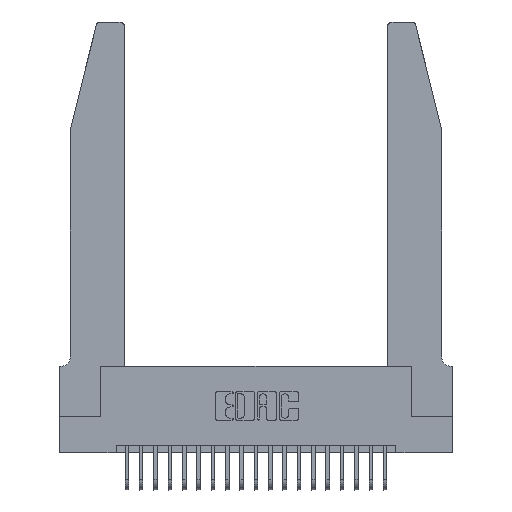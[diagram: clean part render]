
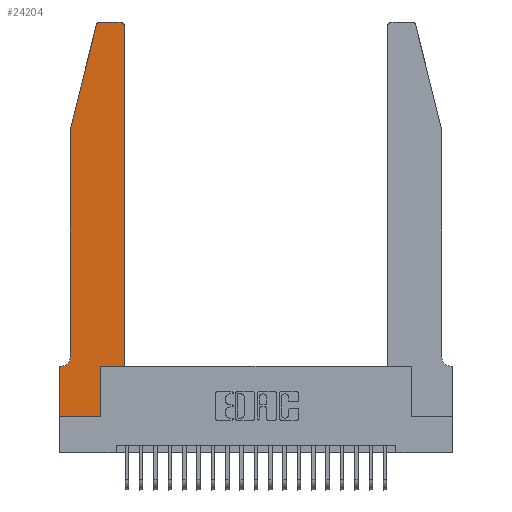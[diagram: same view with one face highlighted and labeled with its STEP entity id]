
A CAD part, top view. The second image highlights one B-rep face of the part: STEP entity #24204.
In plain terms, the highlighted planar face has unit normal (0, 0, 1).
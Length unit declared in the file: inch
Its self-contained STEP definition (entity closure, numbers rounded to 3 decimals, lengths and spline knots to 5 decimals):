
#332 = ORIENTED_EDGE ( 'NONE', *, *, #13802, .T. ) ;
#341 = VERTEX_POINT ( 'NONE', #10353 ) ;
#474 = FACE_OUTER_BOUND ( 'NONE', #6111, .T. ) ;
#601 = EDGE_CURVE ( 'NONE', #7611, #4482, #2556, .T. ) ;
#737 = CARTESIAN_POINT ( 'NONE',  ( 0.0755, 0.42, 0.37 ) ) ;
#818 = ORIENTED_EDGE ( 'NONE', *, *, #16840, .T. ) ;
#1131 = CARTESIAN_POINT ( 'NONE',  ( 0.25487, 2.72718, 0.37 ) ) ;
#1564 = VECTOR ( 'NONE', #19733, 39.37008 ) ;
#1637 = ORIENTED_EDGE ( 'NONE', *, *, #601, .T. ) ;
#1718 = VERTEX_POINT ( 'NONE', #2414 ) ;
#2277 = CARTESIAN_POINT ( 'NONE',  ( 0.284, 2.72, 0.37 ) ) ;
#2356 = DIRECTION ( 'NONE',  ( 1., 0., 0. ) ) ;
#2414 = CARTESIAN_POINT ( 'NONE',  ( 0.4505, 2.72, 0.37 ) ) ;
#2556 = LINE ( 'NONE', #6188, #22008 ) ;
#2585 = EDGE_CURVE ( 'NONE', #13919, #7611, #18211, .T. ) ;
#2730 = LINE ( 'NONE', #12309, #1564 ) ;
#2858 = DIRECTION ( 'NONE',  ( -1., 0., 0. ) ) ;
#3322 = ORIENTED_EDGE ( 'NONE', *, *, #12265, .T. ) ;
#3404 = CARTESIAN_POINT ( 'NONE',  ( 0., 0., 0.37 ) ) ;
#4418 = EDGE_CURVE ( 'NONE', #4507, #13919, #8078, .T. ) ;
#4482 = VERTEX_POINT ( 'NONE', #13182 ) ;
#4507 = VERTEX_POINT ( 'NONE', #5675 ) ;
#4823 = DIRECTION ( 'NONE',  ( 0., 1., 0. ) ) ;
#5077 = ORIENTED_EDGE ( 'NONE', *, *, #18440, .T. ) ;
#5108 = LINE ( 'NONE', #17506, #24265 ) ;
#5464 = DIRECTION ( 'NONE',  ( 0., 0., -1. ) ) ;
#5523 = CARTESIAN_POINT ( 'NONE',  ( 0.4205, 2.72, 0.37 ) ) ;
#5675 = CARTESIAN_POINT ( 'NONE',  ( 0., 0.35, 0.37 ) ) ;
#5890 = EDGE_CURVE ( 'NONE', #4482, #341, #2730, .T. ) ;
#5919 = LINE ( 'NONE', #17060, #17107 ) ;
#6024 = DIRECTION ( 'NONE',  ( -1., 0., 0. ) ) ;
#6111 = EDGE_LOOP ( 'NONE', ( #818, #332, #3322, #20167, #6127, #12152, #15360, #9569, #1637, #6483, #16499, #5077 ) ) ;
#6127 = ORIENTED_EDGE ( 'NONE', *, *, #10615, .T. ) ;
#6188 = CARTESIAN_POINT ( 'NONE',  ( 0.2865, 0.35, 0.37 ) ) ;
#6191 = CARTESIAN_POINT ( 'NONE',  ( 0.0755, 0.35, 0.37 ) ) ;
#6483 = ORIENTED_EDGE ( 'NONE', *, *, #5890, .T. ) ;
#7022 = CARTESIAN_POINT ( 'NONE',  ( 0.0055, 0.42, 0.37 ) ) ;
#7052 = AXIS2_PLACEMENT_3D ( 'NONE', #5523, #13034, #18783 ) ;
#7100 = VECTOR ( 'NONE', #6024, 39.37008 ) ;
#7424 = VERTEX_POINT ( 'NONE', #10633 ) ;
#7493 = VECTOR ( 'NONE', #20188, 39.37008 ) ;
#7611 = VERTEX_POINT ( 'NONE', #9284 ) ;
#7905 = AXIS2_PLACEMENT_3D ( 'NONE', #8267, #14057, #8767 ) ;
#8078 = LINE ( 'NONE', #23388, #7493 ) ;
#8267 = CARTESIAN_POINT ( 'NONE',  ( 0., 0.35, 0.37 ) ) ;
#8580 = CIRCLE ( 'NONE', #24137, 0.03 ) ;
#8668 = CARTESIAN_POINT ( 'NONE',  ( 0.2605, 2.75, 0.37 ) ) ;
#8767 = DIRECTION ( 'NONE',  ( 1., 0., 0. ) ) ;
#9284 = CARTESIAN_POINT ( 'NONE',  ( 0.2865, 0., 0.37 ) ) ;
#9292 = CIRCLE ( 'NONE', #19633, 0.07 ) ;
#9391 = CARTESIAN_POINT ( 'NONE',  ( 0., 0., 0.37 ) ) ;
#9569 = ORIENTED_EDGE ( 'NONE', *, *, #2585, .T. ) ;
#9916 = CARTESIAN_POINT ( 'NONE',  ( 0.284, 2.75, 0.37 ) ) ;
#10353 = CARTESIAN_POINT ( 'NONE',  ( 0.4505, 0.35, 0.37 ) ) ;
#10473 = VERTEX_POINT ( 'NONE', #1131 ) ;
#10475 = DIRECTION ( 'NONE',  ( 0., -1., 0. ) ) ;
#10615 = EDGE_CURVE ( 'NONE', #17444, #22126, #9292, .T. ) ;
#10633 = CARTESIAN_POINT ( 'NONE',  ( 0.0755, 2., 0.37 ) ) ;
#10776 = VERTEX_POINT ( 'NONE', #9916 ) ;
#11362 = DIRECTION ( 'NONE',  ( 1., 0., 0. ) ) ;
#11515 = CIRCLE ( 'NONE', #7052, 0.03 ) ;
#12004 = LINE ( 'NONE', #23497, #17900 ) ;
#12065 = VERTEX_POINT ( 'NONE', #20742 ) ;
#12152 = ORIENTED_EDGE ( 'NONE', *, *, #18036, .T. ) ;
#12265 = EDGE_CURVE ( 'NONE', #10473, #7424, #5108, .T. ) ;
#12309 = CARTESIAN_POINT ( 'NONE',  ( 0.4505, 0.35, 0.37 ) ) ;
#13034 = DIRECTION ( 'NONE',  ( 0., 0., 1. ) ) ;
#13182 = CARTESIAN_POINT ( 'NONE',  ( 0.2865, 0.35, 0.37 ) ) ;
#13802 = EDGE_CURVE ( 'NONE', #10776, #10473, #8580, .T. ) ;
#13919 = VERTEX_POINT ( 'NONE', #3404 ) ;
#14057 = DIRECTION ( 'NONE',  ( 0., 0., 1. ) ) ;
#14195 = LINE ( 'NONE', #6191, #7100 ) ;
#14553 = VECTOR ( 'NONE', #2858, 39.37008 ) ;
#14715 = DIRECTION ( 'NONE',  ( -1., 0., 0. ) ) ;
#15360 = ORIENTED_EDGE ( 'NONE', *, *, #4418, .T. ) ;
#16499 = ORIENTED_EDGE ( 'NONE', *, *, #17964, .T. ) ;
#16840 = EDGE_CURVE ( 'NONE', #12065, #10776, #24297, .T. ) ;
#17060 = CARTESIAN_POINT ( 'NONE',  ( 0.4505, 0.35, 0.37 ) ) ;
#17107 = VECTOR ( 'NONE', #20801, 39.37008 ) ;
#17444 = VERTEX_POINT ( 'NONE', #737 ) ;
#17506 = CARTESIAN_POINT ( 'NONE',  ( 0.0755, 2., 0.37 ) ) ;
#17619 = VECTOR ( 'NONE', #11362, 39.37008 ) ;
#17656 = PLANE ( 'NONE',  #7905 ) ;
#17900 = VECTOR ( 'NONE', #10475, 39.37008 ) ;
#17964 = EDGE_CURVE ( 'NONE', #341, #1718, #5919, .T. ) ;
#18036 = EDGE_CURVE ( 'NONE', #22126, #4507, #14195, .T. ) ;
#18211 = LINE ( 'NONE', #9391, #17619 ) ;
#18440 = EDGE_CURVE ( 'NONE', #1718, #12065, #11515, .T. ) ;
#18644 = CARTESIAN_POINT ( 'NONE',  ( 0.0055, 0.35, 0.37 ) ) ;
#18783 = DIRECTION ( 'NONE',  ( 1., 0., 0. ) ) ;
#19575 = DIRECTION ( 'NONE',  ( -0.239, -0.971, 0. ) ) ;
#19633 = AXIS2_PLACEMENT_3D ( 'NONE', #7022, #5464, #14715 ) ;
#19733 = DIRECTION ( 'NONE',  ( 1., 0., 0. ) ) ;
#20167 = ORIENTED_EDGE ( 'NONE', *, *, #23034, .T. ) ;
#20188 = DIRECTION ( 'NONE',  ( 0., -1., 0. ) ) ;
#20742 = CARTESIAN_POINT ( 'NONE',  ( 0.4205, 2.75, 0.37 ) ) ;
#20801 = DIRECTION ( 'NONE',  ( 0., 1., 0. ) ) ;
#22008 = VECTOR ( 'NONE', #4823, 39.37008 ) ;
#22126 = VERTEX_POINT ( 'NONE', #18644 ) ;
#22933 = DIRECTION ( 'NONE',  ( 0., 0., 1. ) ) ;
#23034 = EDGE_CURVE ( 'NONE', #7424, #17444, #12004, .T. ) ;
#23388 = CARTESIAN_POINT ( 'NONE',  ( 0., 0., 0.37 ) ) ;
#23497 = CARTESIAN_POINT ( 'NONE',  ( 0.0755, 2., 0.37 ) ) ;
#24137 = AXIS2_PLACEMENT_3D ( 'NONE', #2277, #22933, #2356 ) ;
#24204 = ADVANCED_FACE ( 'NONE', ( #474 ), #17656, .T. ) ;
#24265 = VECTOR ( 'NONE', #19575, 39.37008 ) ;
#24297 = LINE ( 'NONE', #8668, #14553 ) ;
